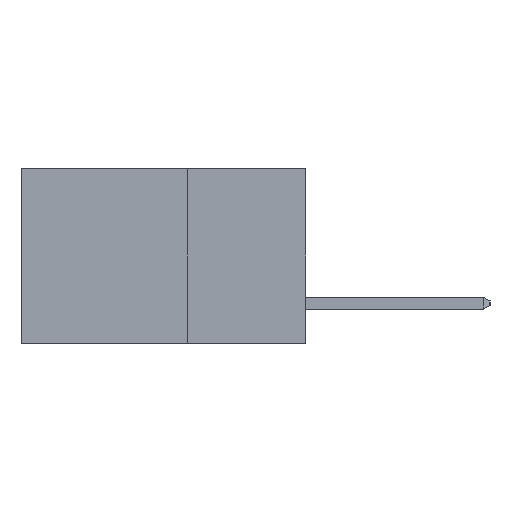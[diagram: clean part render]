
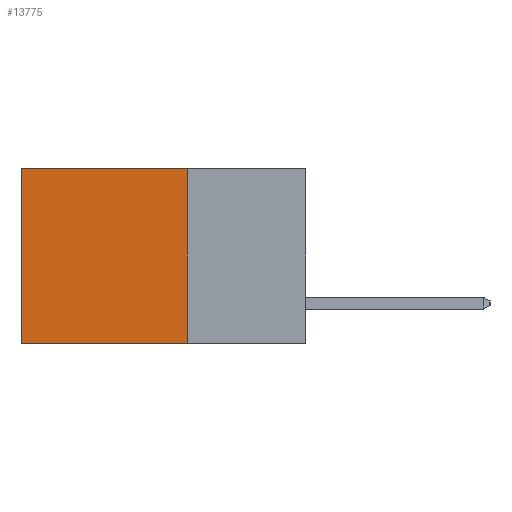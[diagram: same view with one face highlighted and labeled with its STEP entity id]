
A CAD part, left-side view. The second image highlights one B-rep face of the part: STEP entity #13775.
In plain terms, the highlighted planar face has unit normal (-1, 0, 0).
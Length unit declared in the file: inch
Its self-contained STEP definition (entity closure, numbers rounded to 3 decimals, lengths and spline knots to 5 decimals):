
#957 = VERTEX_POINT ( 'NONE', #19407 ) ;
#1859 = LINE ( 'NONE', #2337, #17967 ) ;
#2337 = CARTESIAN_POINT ( 'NONE',  ( 0.298, 0.25, 0. ) ) ;
#2490 = EDGE_CURVE ( 'NONE', #957, #12328, #21036, .T. ) ;
#2748 = AXIS2_PLACEMENT_3D ( 'NONE', #14144, #16284, #3631 ) ;
#2970 = ORIENTED_EDGE ( 'NONE', *, *, #20116, .T. ) ;
#3243 = ORIENTED_EDGE ( 'NONE', *, *, #2490, .F. ) ;
#3631 = DIRECTION ( 'NONE',  ( 0., 0., -1. ) ) ;
#5600 = VERTEX_POINT ( 'NONE', #12207 ) ;
#5831 = CARTESIAN_POINT ( 'NONE',  ( 0.298, 0.6, 0. ) ) ;
#6474 = FACE_OUTER_BOUND ( 'NONE', #15214, .T. ) ;
#6883 = DIRECTION ( 'NONE',  ( 0., 0., -1. ) ) ;
#8649 = DIRECTION ( 'NONE',  ( 0., 0., -1. ) ) ;
#8738 = CARTESIAN_POINT ( 'NONE',  ( 0.298, 0.6, 0. ) ) ;
#8907 = EDGE_CURVE ( 'NONE', #5600, #957, #1859, .T. ) ;
#10748 = EDGE_CURVE ( 'NONE', #22179, #12328, #13976, .T. ) ;
#11237 = ORIENTED_EDGE ( 'NONE', *, *, #8907, .F. ) ;
#12207 = CARTESIAN_POINT ( 'NONE',  ( 0.298, 0.25, 0. ) ) ;
#12328 = VERTEX_POINT ( 'NONE', #19222 ) ;
#13775 = ADVANCED_FACE ( 'NONE', ( #6474 ), #26445, .F. ) ;
#13976 = LINE ( 'NONE', #8738, #24366 ) ;
#14144 = CARTESIAN_POINT ( 'NONE',  ( 0.298, 0.25, 0. ) ) ;
#15214 = EDGE_LOOP ( 'NONE', ( #21925, #3243, #11237, #2970 ) ) ;
#15565 = VECTOR ( 'NONE', #26249, 39.37008 ) ;
#16008 = DIRECTION ( 'NONE',  ( 0., 1., 0. ) ) ;
#16284 = DIRECTION ( 'NONE',  ( 1., 0., 0. ) ) ;
#17967 = VECTOR ( 'NONE', #6883, 39.37008 ) ;
#19222 = CARTESIAN_POINT ( 'NONE',  ( 0.298, 0.6, -0.37 ) ) ;
#19407 = CARTESIAN_POINT ( 'NONE',  ( 0.298, 0.25, -0.37 ) ) ;
#20116 = EDGE_CURVE ( 'NONE', #5600, #22179, #26597, .T. ) ;
#21036 = LINE ( 'NONE', #22069, #15565 ) ;
#21228 = VECTOR ( 'NONE', #16008, 39.37008 ) ;
#21925 = ORIENTED_EDGE ( 'NONE', *, *, #10748, .T. ) ;
#22069 = CARTESIAN_POINT ( 'NONE',  ( 0.298, 0.25, -0.37 ) ) ;
#22179 = VERTEX_POINT ( 'NONE', #5831 ) ;
#22259 = CARTESIAN_POINT ( 'NONE',  ( 0.298, 0.25, 0. ) ) ;
#24366 = VECTOR ( 'NONE', #8649, 39.37008 ) ;
#26249 = DIRECTION ( 'NONE',  ( 0., 1., 0. ) ) ;
#26445 = PLANE ( 'NONE',  #2748 ) ;
#26597 = LINE ( 'NONE', #22259, #21228 ) ;
